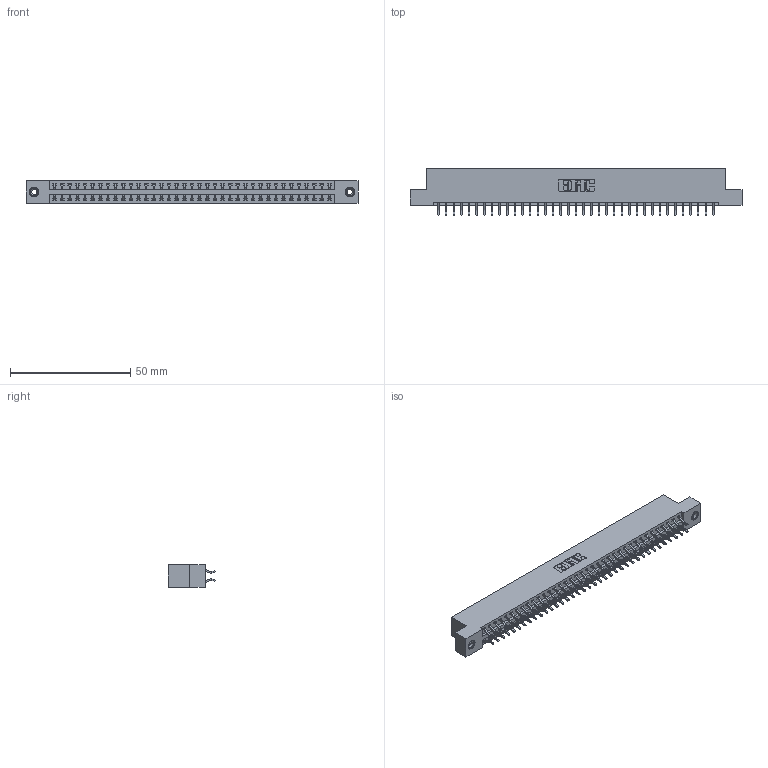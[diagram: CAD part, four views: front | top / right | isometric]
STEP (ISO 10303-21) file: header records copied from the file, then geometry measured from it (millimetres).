
FILE_DESCRIPTION (( 'STEP AP203' ), '1' );
FILE_NAME ('396-074-556-208.STEP', '2019-10-30T20:58:36', ( '' ), ( '' ), 'SwSTEP 2.0', 'SolidWorks 2016', '' );
FILE_SCHEMA (( 'CONFIG_CONTROL_DESIGN' ));
Length unit declared in the file: inch
Products named in the file (4): 346 Part_Flush Mounting Lugs - 0.156 Dia-TI; 396-074-556-208; 345-250-001_345-250-003-102; 345-292-001_556 Tail
Assembly tree (77 placements, depth 2):
  396-074-556-208
    346 Part_Flush Mounting Lugs - 0.156 Dia-TI
    345-292-001_556 Tail  x74
    345-250-001_345-250-003-102  x2
Bounding box: 138.05 x 19.57 x 9.4 mm (x, y, z)
Volume: 13413.2 mm3; surface area: 18310.1 mm2
Topology: 77 solids, 77 shells, 4474 faces, 13267 edges, 8738 vertices
Faces by surface type: plane 2994, cylinder 1464, cone 12, torus 4
Entity records: 26226 total; most frequent: CARTESIAN_POINT 4327, ORIENTED_EDGE 4242, DIRECTION 3879, EDGE_CURVE 2121, LINE 1813, VECTOR 1813, VERTEX_POINT 1408, AXIS2_PLACEMENT_3D 1033
